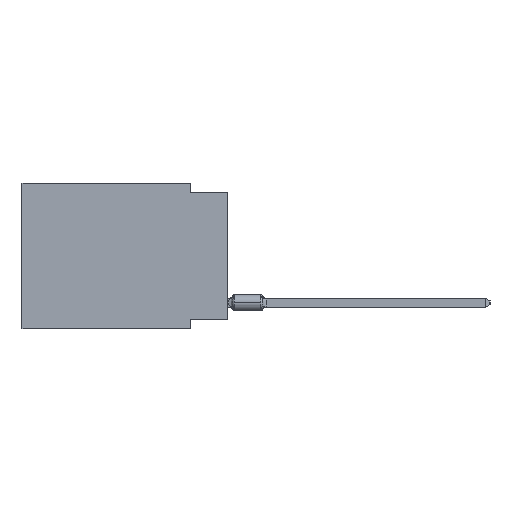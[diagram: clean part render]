
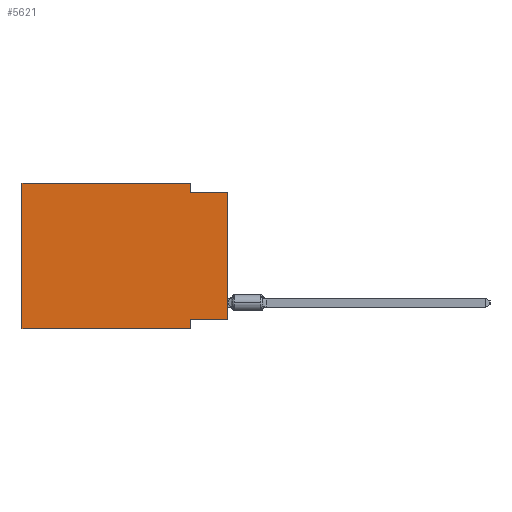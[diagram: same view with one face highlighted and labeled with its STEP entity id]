
A CAD part, left-side view. The second image highlights one B-rep face of the part: STEP entity #5621.
In plain terms, the highlighted planar face has unit normal (-1, 0, 0).
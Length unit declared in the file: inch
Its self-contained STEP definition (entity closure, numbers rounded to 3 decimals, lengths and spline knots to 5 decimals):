
#162 = DIRECTION ( 'NONE',  ( 0., 0., 1. ) ) ;
#767 = LINE ( 'NONE', #25018, #23791 ) ;
#1557 = AXIS2_PLACEMENT_3D ( 'NONE', #2345, #8595, #19668 ) ;
#2136 = DIRECTION ( 'NONE',  ( 0., -1., 0. ) ) ;
#2345 = CARTESIAN_POINT ( 'NONE',  ( 0., 0.55, 0. ) ) ;
#2788 = VECTOR ( 'NONE', #43021, 39.37008 ) ;
#4619 = CARTESIAN_POINT ( 'NONE',  ( 0., 0.55, 0. ) ) ;
#4975 = EDGE_LOOP ( 'NONE', ( #10495, #16324, #9518, #29285, #32506, #39567, #32847, #11309 ) ) ;
#5143 = CARTESIAN_POINT ( 'NONE',  ( 0., 0.1, 0. ) ) ;
#5621 = ADVANCED_FACE ( 'NONE', ( #43927 ), #40231, .F. ) ;
#6180 = CARTESIAN_POINT ( 'NONE',  ( 0., 0.1, -0.365 ) ) ;
#6682 = EDGE_CURVE ( 'NONE', #16156, #19005, #767, .T. ) ;
#7463 = EDGE_CURVE ( 'NONE', #10619, #34931, #32523, .T. ) ;
#7776 = LINE ( 'NONE', #18173, #15828 ) ;
#8595 = DIRECTION ( 'NONE',  ( 1., 0., 0. ) ) ;
#9518 = ORIENTED_EDGE ( 'NONE', *, *, #18635, .F. ) ;
#10495 = ORIENTED_EDGE ( 'NONE', *, *, #32778, .T. ) ;
#10619 = VERTEX_POINT ( 'NONE', #14661 ) ;
#11309 = ORIENTED_EDGE ( 'NONE', *, *, #15370, .F. ) ;
#12134 = VECTOR ( 'NONE', #162, 39.37008 ) ;
#12155 = CARTESIAN_POINT ( 'NONE',  ( 0., 0.55, -0.39 ) ) ;
#13432 = VECTOR ( 'NONE', #13496, 39.37008 ) ;
#13496 = DIRECTION ( 'NONE',  ( 0., 0., 1. ) ) ;
#14661 = CARTESIAN_POINT ( 'NONE',  ( 0., 0.1, -0.025 ) ) ;
#14953 = CARTESIAN_POINT ( 'NONE',  ( 0., 0., -0.025 ) ) ;
#15370 = EDGE_CURVE ( 'NONE', #29336, #16156, #7776, .T. ) ;
#15828 = VECTOR ( 'NONE', #35962, 39.37008 ) ;
#16156 = VERTEX_POINT ( 'NONE', #6180 ) ;
#16324 = ORIENTED_EDGE ( 'NONE', *, *, #7463, .F. ) ;
#17294 = VERTEX_POINT ( 'NONE', #4619 ) ;
#17796 = CARTESIAN_POINT ( 'NONE',  ( 0., 0.1, -0.39 ) ) ;
#18173 = CARTESIAN_POINT ( 'NONE',  ( 0., 0., -0.365 ) ) ;
#18635 = EDGE_CURVE ( 'NONE', #36173, #10619, #36788, .T. ) ;
#19005 = VERTEX_POINT ( 'NONE', #17796 ) ;
#19668 = DIRECTION ( 'NONE',  ( 0., 0., -1. ) ) ;
#20144 = CARTESIAN_POINT ( 'NONE',  ( 0., 0., -0.025 ) ) ;
#21053 = VECTOR ( 'NONE', #33010, 39.37008 ) ;
#22908 = CARTESIAN_POINT ( 'NONE',  ( 0., 0.55, -0.39 ) ) ;
#23461 = VECTOR ( 'NONE', #29045, 39.37008 ) ;
#23791 = VECTOR ( 'NONE', #39322, 39.37008 ) ;
#25018 = CARTESIAN_POINT ( 'NONE',  ( 0., 0.1, -0.39 ) ) ;
#25354 = VERTEX_POINT ( 'NONE', #12155 ) ;
#25384 = CARTESIAN_POINT ( 'NONE',  ( 0., 0., -0.365 ) ) ;
#26388 = LINE ( 'NONE', #22908, #26593 ) ;
#26593 = VECTOR ( 'NONE', #2136, 39.37008 ) ;
#27590 = CARTESIAN_POINT ( 'NONE',  ( 0., 0.55, 0. ) ) ;
#29045 = DIRECTION ( 'NONE',  ( 0., -1., 0. ) ) ;
#29285 = ORIENTED_EDGE ( 'NONE', *, *, #35542, .F. ) ;
#29336 = VERTEX_POINT ( 'NONE', #25384 ) ;
#29905 = CARTESIAN_POINT ( 'NONE',  ( 0., 0.1, 0. ) ) ;
#32506 = ORIENTED_EDGE ( 'NONE', *, *, #38084, .F. ) ;
#32523 = LINE ( 'NONE', #14953, #23461 ) ;
#32778 = EDGE_CURVE ( 'NONE', #29336, #34931, #42427, .T. ) ;
#32847 = ORIENTED_EDGE ( 'NONE', *, *, #6682, .F. ) ;
#33010 = DIRECTION ( 'NONE',  ( 0., -1., 0. ) ) ;
#34931 = VERTEX_POINT ( 'NONE', #20144 ) ;
#34977 = LINE ( 'NONE', #27590, #13432 ) ;
#35038 = CARTESIAN_POINT ( 'NONE',  ( 0., 0., 0. ) ) ;
#35542 = EDGE_CURVE ( 'NONE', #17294, #36173, #40152, .T. ) ;
#35962 = DIRECTION ( 'NONE',  ( 0., 1., 0. ) ) ;
#36173 = VERTEX_POINT ( 'NONE', #29905 ) ;
#36535 = EDGE_CURVE ( 'NONE', #25354, #19005, #26388, .T. ) ;
#36788 = LINE ( 'NONE', #5143, #2788 ) ;
#36912 = CARTESIAN_POINT ( 'NONE',  ( 0., 0.55, 0. ) ) ;
#38084 = EDGE_CURVE ( 'NONE', #25354, #17294, #34977, .T. ) ;
#39322 = DIRECTION ( 'NONE',  ( 0., 0., -1. ) ) ;
#39567 = ORIENTED_EDGE ( 'NONE', *, *, #36535, .T. ) ;
#40152 = LINE ( 'NONE', #36912, #21053 ) ;
#40231 = PLANE ( 'NONE',  #1557 ) ;
#42427 = LINE ( 'NONE', #35038, #12134 ) ;
#43021 = DIRECTION ( 'NONE',  ( 0., 0., -1. ) ) ;
#43927 = FACE_OUTER_BOUND ( 'NONE', #4975, .T. ) ;
